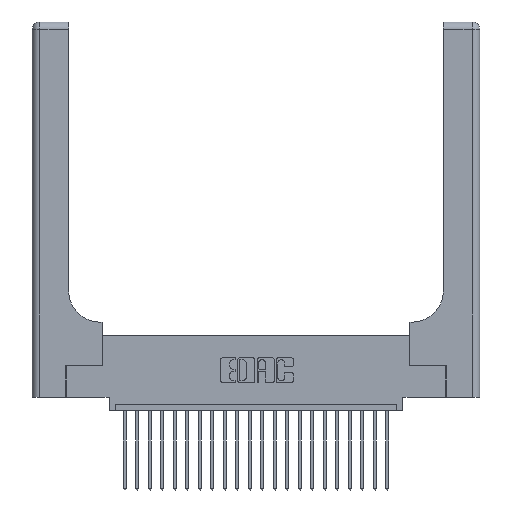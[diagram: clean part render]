
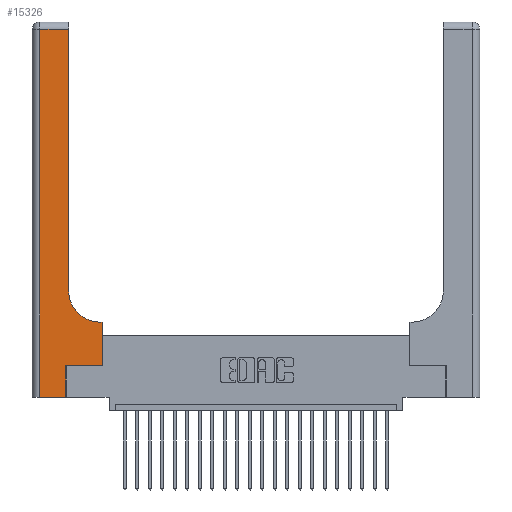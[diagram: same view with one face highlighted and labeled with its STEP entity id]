
A CAD part, top view. The second image highlights one B-rep face of the part: STEP entity #15326.
In plain terms, the highlighted planar face has unit normal (0, 0, 1).
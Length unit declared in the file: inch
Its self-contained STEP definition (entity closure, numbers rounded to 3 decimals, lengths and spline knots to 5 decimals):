
#123 = VERTEX_POINT ( 'NONE', #11263 ) ;
#1248 = CARTESIAN_POINT ( 'NONE',  ( 0.5415, 0.6, 0.37 ) ) ;
#1263 = DIRECTION ( 'NONE',  ( 0., 0., -1. ) ) ;
#1280 = VERTEX_POINT ( 'NONE', #11731 ) ;
#1552 = EDGE_CURVE ( 'NONE', #10957, #4537, #11860, .T. ) ;
#1747 = AXIS2_PLACEMENT_3D ( 'NONE', #16237, #1263, #18120 ) ;
#2424 = PLANE ( 'NONE',  #11743 ) ;
#2451 = EDGE_LOOP ( 'NONE', ( #17455, #3716, #13468, #3122, #11739, #17149, #9468, #14476, #3661 ) ) ;
#2760 = LINE ( 'NONE', #19581, #21470 ) ;
#2872 = CARTESIAN_POINT ( 'NONE',  ( 0.269, 0., 0.37 ) ) ;
#3122 = ORIENTED_EDGE ( 'NONE', *, *, #4183, .T. ) ;
#3603 = LINE ( 'NONE', #18833, #15186 ) ;
#3661 = ORIENTED_EDGE ( 'NONE', *, *, #5099, .T. ) ;
#3716 = ORIENTED_EDGE ( 'NONE', *, *, #1552, .T. ) ;
#4183 = EDGE_CURVE ( 'NONE', #123, #7121, #3603, .T. ) ;
#4537 = VERTEX_POINT ( 'NONE', #4857 ) ;
#4857 = CARTESIAN_POINT ( 'NONE',  ( 0.06, 2.94, 0.37 ) ) ;
#5099 = EDGE_CURVE ( 'NONE', #21978, #14937, #14889, .T. ) ;
#6043 = DIRECTION ( 'NONE',  ( -1., 0., 0. ) ) ;
#6068 = CARTESIAN_POINT ( 'NONE',  ( 0.2915, 3., 0.37 ) ) ;
#6126 = VECTOR ( 'NONE', #11482, 39.37008 ) ;
#6228 = VERTEX_POINT ( 'NONE', #17299 ) ;
#6676 = DIRECTION ( 'NONE',  ( -1., 0., 0. ) ) ;
#7121 = VERTEX_POINT ( 'NONE', #15313 ) ;
#7334 = VERTEX_POINT ( 'NONE', #13454 ) ;
#7741 = VECTOR ( 'NONE', #11154, 39.37008 ) ;
#8378 = LINE ( 'NONE', #2872, #20826 ) ;
#9468 = ORIENTED_EDGE ( 'NONE', *, *, #22649, .T. ) ;
#9543 = EDGE_CURVE ( 'NONE', #7121, #6228, #8378, .T. ) ;
#9583 = DIRECTION ( 'NONE',  ( 1., 0., 0. ) ) ;
#10957 = VERTEX_POINT ( 'NONE', #11533 ) ;
#11008 = CARTESIAN_POINT ( 'NONE',  ( 0.2915, 0.85, 0.37 ) ) ;
#11154 = DIRECTION ( 'NONE',  ( 0., 1., 0. ) ) ;
#11263 = CARTESIAN_POINT ( 'NONE',  ( 0.06, 0., 0.37 ) ) ;
#11482 = DIRECTION ( 'NONE',  ( 0., -1., 0. ) ) ;
#11533 = CARTESIAN_POINT ( 'NONE',  ( 0.2915, 2.94, 0.37 ) ) ;
#11731 = CARTESIAN_POINT ( 'NONE',  ( 0.5585, 0.25, 0.37 ) ) ;
#11739 = ORIENTED_EDGE ( 'NONE', *, *, #9543, .T. ) ;
#11743 = AXIS2_PLACEMENT_3D ( 'NONE', #19517, #11750, #6043 ) ;
#11750 = DIRECTION ( 'NONE',  ( 0., 0., -1. ) ) ;
#11860 = LINE ( 'NONE', #18005, #16313 ) ;
#12560 = VECTOR ( 'NONE', #20590, 39.37008 ) ;
#12785 = LINE ( 'NONE', #20498, #7741 ) ;
#13454 = CARTESIAN_POINT ( 'NONE',  ( 0.5585, 0.6, 0.37 ) ) ;
#13468 = ORIENTED_EDGE ( 'NONE', *, *, #17634, .T. ) ;
#13591 = VECTOR ( 'NONE', #15671, 39.37008 ) ;
#13860 = EDGE_CURVE ( 'NONE', #7334, #21978, #2760, .T. ) ;
#14476 = ORIENTED_EDGE ( 'NONE', *, *, #13860, .T. ) ;
#14608 = EDGE_CURVE ( 'NONE', #6228, #1280, #21448, .T. ) ;
#14889 = CIRCLE ( 'NONE', #1747, 0.25 ) ;
#14937 = VERTEX_POINT ( 'NONE', #11008 ) ;
#15186 = VECTOR ( 'NONE', #9583, 39.37008 ) ;
#15313 = CARTESIAN_POINT ( 'NONE',  ( 0.269, 0., 0.37 ) ) ;
#15326 = ADVANCED_FACE ( 'NONE', ( #16296 ), #2424, .F. ) ;
#15671 = DIRECTION ( 'NONE',  ( 0., 1., 0. ) ) ;
#16237 = CARTESIAN_POINT ( 'NONE',  ( 0.5415, 0.85, 0.37 ) ) ;
#16296 = FACE_OUTER_BOUND ( 'NONE', #2451, .T. ) ;
#16313 = VECTOR ( 'NONE', #6676, 39.37008 ) ;
#16544 = CARTESIAN_POINT ( 'NONE',  ( 0.269, 0.25, 0.37 ) ) ;
#17099 = CARTESIAN_POINT ( 'NONE',  ( 0.06, 3., 0.37 ) ) ;
#17149 = ORIENTED_EDGE ( 'NONE', *, *, #14608, .T. ) ;
#17299 = CARTESIAN_POINT ( 'NONE',  ( 0.269, 0.25, 0.37 ) ) ;
#17455 = ORIENTED_EDGE ( 'NONE', *, *, #24005, .T. ) ;
#17634 = EDGE_CURVE ( 'NONE', #4537, #123, #17658, .T. ) ;
#17658 = LINE ( 'NONE', #17099, #6126 ) ;
#18005 = CARTESIAN_POINT ( 'NONE',  ( 0., 2.94, 0.37 ) ) ;
#18120 = DIRECTION ( 'NONE',  ( 1., 0., 0. ) ) ;
#18833 = CARTESIAN_POINT ( 'NONE',  ( 0., 0., 0.37 ) ) ;
#19517 = CARTESIAN_POINT ( 'NONE',  ( 0., 3., 0.37 ) ) ;
#19581 = CARTESIAN_POINT ( 'NONE',  ( 0.2915, 0.6, 0.37 ) ) ;
#20498 = CARTESIAN_POINT ( 'NONE',  ( 0.5585, 0.25, 0.37 ) ) ;
#20590 = DIRECTION ( 'NONE',  ( 1., 0., 0. ) ) ;
#20826 = VECTOR ( 'NONE', #21886, 39.37008 ) ;
#21448 = LINE ( 'NONE', #16544, #12560 ) ;
#21470 = VECTOR ( 'NONE', #21744, 39.37008 ) ;
#21744 = DIRECTION ( 'NONE',  ( -1., 0., 0. ) ) ;
#21886 = DIRECTION ( 'NONE',  ( 0., 1., 0. ) ) ;
#21978 = VERTEX_POINT ( 'NONE', #1248 ) ;
#22649 = EDGE_CURVE ( 'NONE', #1280, #7334, #12785, .T. ) ;
#23615 = LINE ( 'NONE', #6068, #13591 ) ;
#24005 = EDGE_CURVE ( 'NONE', #14937, #10957, #23615, .T. ) ;
